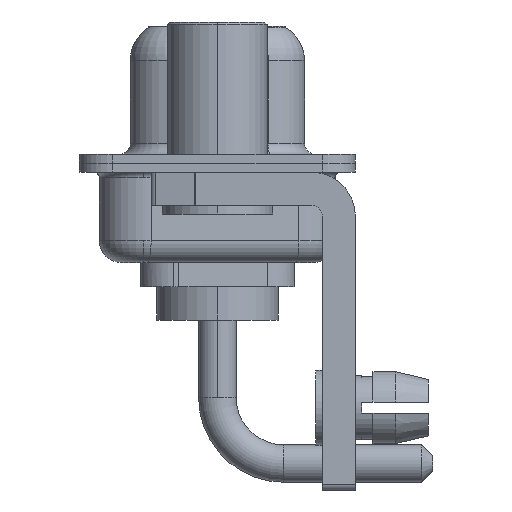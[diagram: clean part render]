
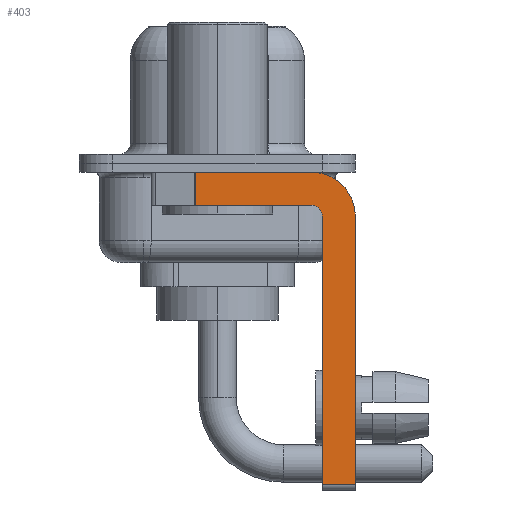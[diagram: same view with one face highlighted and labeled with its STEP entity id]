
A CAD part, left-side view. The second image highlights one B-rep face of the part: STEP entity #403.
In plain terms, the highlighted planar face has unit normal (-1, 0, 0).
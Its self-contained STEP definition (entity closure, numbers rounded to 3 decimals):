
#226 = ORIENTED_EDGE ( 'NONE', *, *, #1396, .F. ) ;
#403 = ADVANCED_FACE ( 'NONE', ( #10673 ), #13494, .F. ) ;
#614 = EDGE_CURVE ( 'NONE', #3692, #9208, #1213, .T. ) ;
#794 = DIRECTION ( 'NONE',  ( 0., 0., -1. ) ) ;
#873 = ORIENTED_EDGE ( 'NONE', *, *, #12434, .F. ) ;
#1049 = DIRECTION ( 'NONE',  ( 0., 0., -1. ) ) ;
#1154 = VECTOR ( 'NONE', #14627, 1000. ) ;
#1199 = CARTESIAN_POINT ( 'NONE',  ( -2.9, -6.25, -14.55 ) ) ;
#1213 = LINE ( 'NONE', #11346, #4487 ) ;
#1248 = ORIENTED_EDGE ( 'NONE', *, *, #11019, .F. ) ;
#1396 = EDGE_CURVE ( 'NONE', #10517, #8967, #16483, .T. ) ;
#1405 = CARTESIAN_POINT ( 'NONE',  ( -2.9, -4.25, -1.9 ) ) ;
#1466 = DIRECTION ( 'NONE',  ( 0., 1., 0. ) ) ;
#1565 = CARTESIAN_POINT ( 'NONE',  ( -2.9, -4.25, -0.4 ) ) ;
#1682 = CARTESIAN_POINT ( 'NONE',  ( -2.9, -4.25, -14.55 ) ) ;
#1824 = VERTEX_POINT ( 'NONE', #6321 ) ;
#2948 = CARTESIAN_POINT ( 'NONE',  ( -2.9, -4.25, -2.4 ) ) ;
#3023 = CARTESIAN_POINT ( 'NONE',  ( -2.9, -4.75, -14.8 ) ) ;
#3452 = EDGE_CURVE ( 'NONE', #1824, #11812, #16062, .T. ) ;
#3557 = VECTOR ( 'NONE', #16116, 1000. ) ;
#3560 = EDGE_CURVE ( 'NONE', #6491, #8967, #9259, .T. ) ;
#3692 = VERTEX_POINT ( 'NONE', #8167 ) ;
#4043 = EDGE_LOOP ( 'NONE', ( #1248, #6099, #5339, #6718, #873, #5864, #226, #12070 ) ) ;
#4206 = CIRCLE ( 'NONE', #12906, 2. ) ;
#4487 = VECTOR ( 'NONE', #1049, 1000. ) ;
#4686 = CARTESIAN_POINT ( 'NONE',  ( -2.9, 0.978, -1.9 ) ) ;
#4718 = DIRECTION ( 'NONE',  ( 1., 0., 0. ) ) ;
#5185 = CARTESIAN_POINT ( 'NONE',  ( -2.9, -4.25, -2.4 ) ) ;
#5339 = ORIENTED_EDGE ( 'NONE', *, *, #8351, .F. ) ;
#5864 = ORIENTED_EDGE ( 'NONE', *, *, #3560, .T. ) ;
#6099 = ORIENTED_EDGE ( 'NONE', *, *, #614, .T. ) ;
#6301 = AXIS2_PLACEMENT_3D ( 'NONE', #10840, #4718, #794 ) ;
#6319 = DIRECTION ( 'NONE',  ( -1., 0., 0. ) ) ;
#6321 = CARTESIAN_POINT ( 'NONE',  ( -2.9, -4.75, -2.4 ) ) ;
#6417 = CARTESIAN_POINT ( 'NONE',  ( -2.9, -6.25, -2.4 ) ) ;
#6491 = VERTEX_POINT ( 'NONE', #10792 ) ;
#6718 = ORIENTED_EDGE ( 'NONE', *, *, #3452, .F. ) ;
#8167 = CARTESIAN_POINT ( 'NONE',  ( -2.9, 0.978, -0.4 ) ) ;
#8351 = EDGE_CURVE ( 'NONE', #11812, #9208, #14249, .T. ) ;
#8466 = CARTESIAN_POINT ( 'NONE',  ( -2.9, -6.25, -2.4 ) ) ;
#8967 = VERTEX_POINT ( 'NONE', #1199 ) ;
#9092 = DIRECTION ( 'NONE',  ( 0., 0., -1. ) ) ;
#9208 = VERTEX_POINT ( 'NONE', #4686 ) ;
#9259 = LINE ( 'NONE', #1682, #14283 ) ;
#10517 = VERTEX_POINT ( 'NONE', #8466 ) ;
#10673 = FACE_OUTER_BOUND ( 'NONE', #4043, .T. ) ;
#10792 = CARTESIAN_POINT ( 'NONE',  ( -2.9, -4.75, -14.55 ) ) ;
#10840 = CARTESIAN_POINT ( 'NONE',  ( -2.9, -4.25, -2.4 ) ) ;
#10856 = LINE ( 'NONE', #3023, #1154 ) ;
#11019 = EDGE_CURVE ( 'NONE', #3692, #12917, #14919, .T. ) ;
#11346 = CARTESIAN_POINT ( 'NONE',  ( -2.9, 0.978, -1.9 ) ) ;
#11812 = VERTEX_POINT ( 'NONE', #1405 ) ;
#12070 = ORIENTED_EDGE ( 'NONE', *, *, #14346, .F. ) ;
#12349 = CARTESIAN_POINT ( 'NONE',  ( -2.9, 3., -0.4 ) ) ;
#12434 = EDGE_CURVE ( 'NONE', #6491, #1824, #10856, .T. ) ;
#12809 = CARTESIAN_POINT ( 'NONE',  ( -2.9, -4.25, -1.9 ) ) ;
#12906 = AXIS2_PLACEMENT_3D ( 'NONE', #2948, #13177, #9092 ) ;
#12917 = VERTEX_POINT ( 'NONE', #1565 ) ;
#13177 = DIRECTION ( 'NONE',  ( 1., 0., 0. ) ) ;
#13494 = PLANE ( 'NONE',  #6301 ) ;
#14213 = DIRECTION ( 'NONE',  ( 0., 0., 1. ) ) ;
#14249 = LINE ( 'NONE', #12809, #16814 ) ;
#14283 = VECTOR ( 'NONE', #15998, 1000. ) ;
#14346 = EDGE_CURVE ( 'NONE', #12917, #10517, #4206, .T. ) ;
#14627 = DIRECTION ( 'NONE',  ( 0., 0., 1. ) ) ;
#14919 = LINE ( 'NONE', #12349, #3557 ) ;
#14938 = VECTOR ( 'NONE', #15591, 1000. ) ;
#14974 = AXIS2_PLACEMENT_3D ( 'NONE', #5185, #6319, #14213 ) ;
#15591 = DIRECTION ( 'NONE',  ( 0., 0., -1. ) ) ;
#15998 = DIRECTION ( 'NONE',  ( 0., -1., 0. ) ) ;
#16062 = CIRCLE ( 'NONE', #14974, 0.5 ) ;
#16116 = DIRECTION ( 'NONE',  ( 0., -1., 0. ) ) ;
#16483 = LINE ( 'NONE', #6417, #14938 ) ;
#16814 = VECTOR ( 'NONE', #1466, 1000. ) ;
